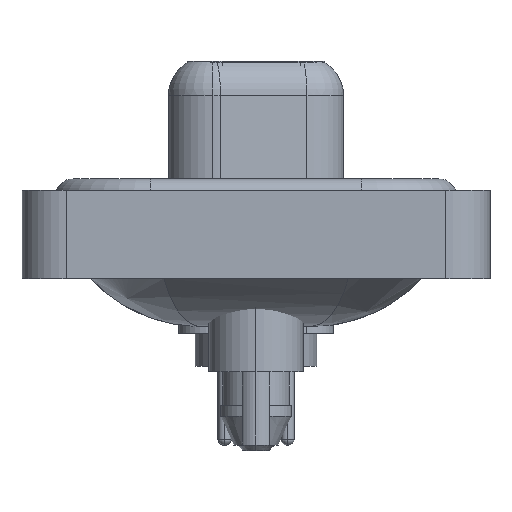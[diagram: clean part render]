
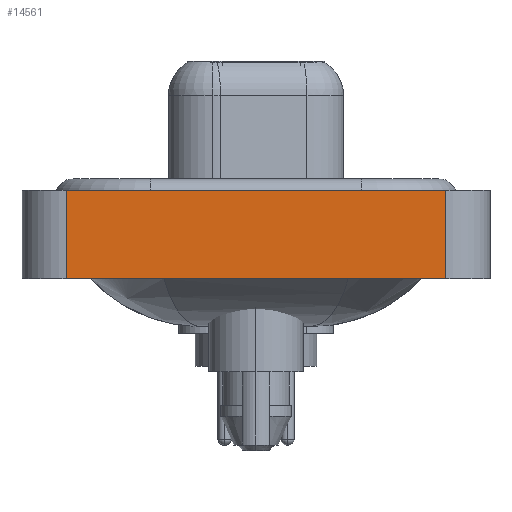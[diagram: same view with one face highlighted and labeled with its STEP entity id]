
A CAD part, left-side view. The second image highlights one B-rep face of the part: STEP entity #14561.
In plain terms, the highlighted planar face has unit normal (-1, 0, 0).
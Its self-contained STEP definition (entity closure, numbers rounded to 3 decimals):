
#176 = DIRECTION ( 'NONE',  ( 0., 0., 1. ) ) ;
#289 = DIRECTION ( 'NONE',  ( 0., -1., 0. ) ) ;
#664 = VERTEX_POINT ( 'NONE', #13050 ) ;
#750 = EDGE_CURVE ( 'NONE', #12354, #13593, #18298, .T. ) ;
#1600 = VERTEX_POINT ( 'NONE', #4212 ) ;
#2773 = DIRECTION ( 'NONE',  ( 0., 0., 1. ) ) ;
#2993 = VECTOR ( 'NONE', #289, 1000. ) ;
#3596 = EDGE_CURVE ( 'NONE', #1600, #664, #11930, .T. ) ;
#3633 = LINE ( 'NONE', #12346, #2993 ) ;
#4212 = CARTESIAN_POINT ( 'NONE',  ( -7.3, 8.55, -3.6 ) ) ;
#4872 = CARTESIAN_POINT ( 'NONE',  ( -7.3, -8.55, -3.6 ) ) ;
#5992 = CARTESIAN_POINT ( 'NONE',  ( -7.3, -8.55, -3.6 ) ) ;
#7315 = LINE ( 'NONE', #18985, #19230 ) ;
#8379 = CARTESIAN_POINT ( 'NONE',  ( -7.3, 8.55, -3.6 ) ) ;
#8505 = AXIS2_PLACEMENT_3D ( 'NONE', #5992, #9305, #16416 ) ;
#9247 = CARTESIAN_POINT ( 'NONE',  ( -7.3, -8.55, -3.6 ) ) ;
#9305 = DIRECTION ( 'NONE',  ( -1., 0., 0. ) ) ;
#10143 = VECTOR ( 'NONE', #176, 1000. ) ;
#10355 = VECTOR ( 'NONE', #2773, 1000. ) ;
#10863 = PLANE ( 'NONE',  #8505 ) ;
#11930 = LINE ( 'NONE', #8379, #10143 ) ;
#12145 = ORIENTED_EDGE ( 'NONE', *, *, #3596, .F. ) ;
#12346 = CARTESIAN_POINT ( 'NONE',  ( -7.3, -8.55, -3.6 ) ) ;
#12347 = CARTESIAN_POINT ( 'NONE',  ( -7.3, -8.55, 0.4 ) ) ;
#12354 = VERTEX_POINT ( 'NONE', #9247 ) ;
#12967 = EDGE_LOOP ( 'NONE', ( #17494, #18988, #12145, #15504 ) ) ;
#13050 = CARTESIAN_POINT ( 'NONE',  ( -7.3, 8.55, 0.4 ) ) ;
#13593 = VERTEX_POINT ( 'NONE', #12347 ) ;
#14561 = ADVANCED_FACE ( 'NONE', ( #16091 ), #10863, .T. ) ;
#15504 = ORIENTED_EDGE ( 'NONE', *, *, #18698, .T. ) ;
#15751 = EDGE_CURVE ( 'NONE', #664, #13593, #7315, .T. ) ;
#16091 = FACE_OUTER_BOUND ( 'NONE', #12967, .T. ) ;
#16416 = DIRECTION ( 'NONE',  ( 0., 0., 1. ) ) ;
#17494 = ORIENTED_EDGE ( 'NONE', *, *, #750, .T. ) ;
#18298 = LINE ( 'NONE', #4872, #10355 ) ;
#18698 = EDGE_CURVE ( 'NONE', #1600, #12354, #3633, .T. ) ;
#18985 = CARTESIAN_POINT ( 'NONE',  ( -7.3, -8.55, 0.4 ) ) ;
#18988 = ORIENTED_EDGE ( 'NONE', *, *, #15751, .F. ) ;
#19200 = DIRECTION ( 'NONE',  ( 0., -1., 0. ) ) ;
#19230 = VECTOR ( 'NONE', #19200, 1000. ) ;
